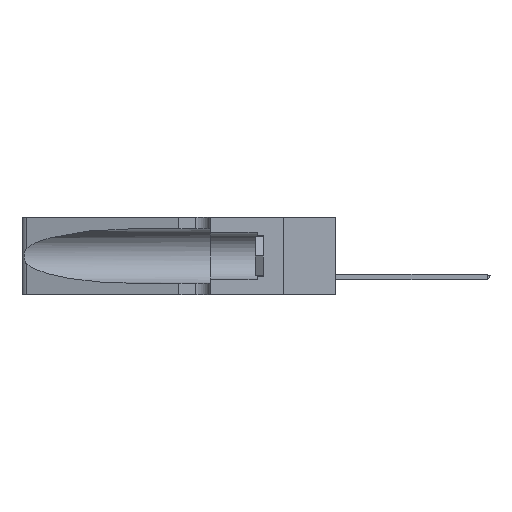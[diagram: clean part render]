
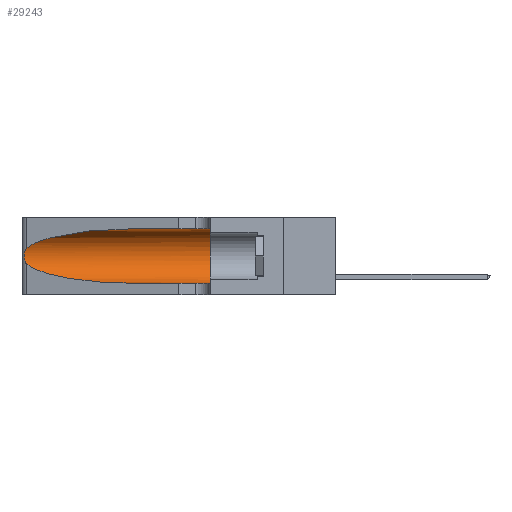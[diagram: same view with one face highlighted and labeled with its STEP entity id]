
A CAD part, left-side view. The second image highlights one B-rep face of the part: STEP entity #29243.
In plain terms, the highlighted cylindrical face has radius 3.308 mm (diameter 6.617 mm), a partial arc.
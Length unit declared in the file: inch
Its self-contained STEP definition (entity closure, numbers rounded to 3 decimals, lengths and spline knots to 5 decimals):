
#1858 = CARTESIAN_POINT ( 'NONE',  ( 0.25487, 1.22718, 0.22369 ) ) ;
#1922 = CARTESIAN_POINT ( 'NONE',  ( 0.2373, 1.15595, 0.08982 ) ) ;
#2333 = CARTESIAN_POINT ( 'NONE',  ( 0.1305, 0.72297, 0.05475 ) ) ;
#2973 = DIRECTION ( 'NONE',  ( 0., -1., 0. ) ) ;
#5405 = CARTESIAN_POINT ( 'NONE',  ( 0.25487, 1.22718, 0.14631 ) ) ;
#5697 = CARTESIAN_POINT ( 'NONE',  ( 0.25854, 1.2359, 0.20912 ) ) ;
#5818 = CIRCLE ( 'NONE', #12054, 0.13025 ) ;
#7218 = DIRECTION ( 'NONE',  ( 0., 0., 1. ) ) ;
#7239 = DIRECTION ( 'NONE',  ( 0., -1., 0. ) ) ;
#7393 = EDGE_CURVE ( 'NONE', #26052, #35483, #23787, .T. ) ;
#8834 = EDGE_CURVE ( 'NONE', #19129, #9179, #31826, .T. ) ;
#8883 = CARTESIAN_POINT ( 'NONE',  ( 0.26075, 1.23896, 0.178 ) ) ;
#9179 = VERTEX_POINT ( 'NONE', #26367 ) ;
#9189 = ORIENTED_EDGE ( 'NONE', *, *, #22624, .T. ) ;
#9213 = CARTESIAN_POINT ( 'NONE',  ( 0.1305, 1.61858, 0.31525 ) ) ;
#9993 = CARTESIAN_POINT ( 'NONE',  ( 0.1305, 0.35, 0.185 ) ) ;
#10041 = ORIENTED_EDGE ( 'NONE', *, *, #10810, .F. ) ;
#10499 = EDGE_LOOP ( 'NONE', ( #9189, #23590, #22509, #21826, #10041, #40537 ) ) ;
#10810 = EDGE_CURVE ( 'NONE', #35483, #9179, #5818, .T. ) ;
#11647 = AXIS2_PLACEMENT_3D ( 'NONE', #26036, #7239, #26172 ) ;
#12054 = AXIS2_PLACEMENT_3D ( 'NONE', #9993, #32404, #7218 ) ;
#12068 = CARTESIAN_POINT ( 'NONE',  ( 0.25487, 1.22718, 0.22369 ) ) ;
#12842 = CARTESIAN_POINT ( 'NONE',  ( 0.1305, 0.35, 0.31525 ) ) ;
#12976 = CARTESIAN_POINT ( 'NONE',  ( 0.25487, 1.22718, 0.22369 ) ) ;
#15399 = CARTESIAN_POINT ( 'NONE',  ( 0.25639, 1.23184, 0.21858 ) ) ;
#15544 = CARTESIAN_POINT ( 'NONE',  ( 0.25555, 1.22994, 0.2215 ) ) ;
#15869 = CARTESIAN_POINT ( 'NONE',  ( 0.1305, 1.61858, 0.05475 ) ) ;
#16660 = EDGE_CURVE ( 'NONE', #23271, #27142, #37375, .T. ) ;
#17278 = CARTESIAN_POINT ( 'NONE',  ( 0.1305, 0.72297, 0.31525 ) ) ;
#17687 = CARTESIAN_POINT ( 'NONE',  ( 0.2373, 1.15595, 0.28018 ) ) ;
#17763 = CARTESIAN_POINT ( 'NONE',  ( 0.25487, 1.22718, 0.14631 ) ) ;
#17846 = VECTOR ( 'NONE', #34708, 39.37008 ) ;
#18180 = CARTESIAN_POINT ( 'NONE',  ( 0.25787, 1.23484, 0.2124 ) ) ;
#18328 = CARTESIAN_POINT ( 'NONE',  ( 0.25856, 1.23593, 0.16098 ) ) ;
#18611 = CARTESIAN_POINT ( 'NONE',  ( 0.25487, 1.22718, 0.14631 ) ) ;
#19129 = VERTEX_POINT ( 'NONE', #24128 ) ;
#20222 = CARTESIAN_POINT ( 'NONE',  ( 0.1305, 0.72297, 0.31525 ) ) ;
#21520 = CARTESIAN_POINT ( 'NONE',  ( 0.25639, 1.23186, 0.15144 ) ) ;
#21826 = ORIENTED_EDGE ( 'NONE', *, *, #8834, .T. ) ;
#22342 = VECTOR ( 'NONE', #2973, 39.37008 ) ;
#22509 = ORIENTED_EDGE ( 'NONE', *, *, #26175, .T. ) ;
#22624 = EDGE_CURVE ( 'NONE', #26052, #23271, #36076, .T. ) ;
#23271 = VERTEX_POINT ( 'NONE', #12976 ) ;
#23590 = ORIENTED_EDGE ( 'NONE', *, *, #16660, .T. ) ;
#23787 = LINE ( 'NONE', #9213, #17846 ) ;
#23802 =( BOUNDED_CURVE ( )  B_SPLINE_CURVE ( 3, ( #5405, #1922, #34059, #2333 ),
 .UNSPECIFIED., .F., .T. ) 
 B_SPLINE_CURVE_WITH_KNOTS ( ( 4, 4 ),
 ( 3.44316, 4.71239 ),
 .UNSPECIFIED. ) 
 CURVE ( )  GEOMETRIC_REPRESENTATION_ITEM ( )  RATIONAL_B_SPLINE_CURVE ( ( 1., 0.87, 0.87, 1. ) ) 
 REPRESENTATION_ITEM ( '' )  );
#24128 = CARTESIAN_POINT ( 'NONE',  ( 0.1305, 0.72297, 0.05475 ) ) ;
#26036 = CARTESIAN_POINT ( 'NONE',  ( 0.1305, 1.61858, 0.185 ) ) ;
#26052 = VERTEX_POINT ( 'NONE', #20222 ) ;
#26172 = DIRECTION ( 'NONE',  ( 0., 0., -1. ) ) ;
#26175 = EDGE_CURVE ( 'NONE', #27142, #19129, #23802, .T. ) ;
#26367 = CARTESIAN_POINT ( 'NONE',  ( 0.1305, 0.35, 0.05475 ) ) ;
#27142 = VERTEX_POINT ( 'NONE', #17763 ) ;
#27181 = CARTESIAN_POINT ( 'NONE',  ( 0.18966, 0.96281, 0.31525 ) ) ;
#27805 = CARTESIAN_POINT ( 'NONE',  ( 0.26018, 1.23835, 0.19895 ) ) ;
#29243 = ADVANCED_FACE ( 'NONE', ( #38303 ), #31329, .F. ) ;
#30997 = CARTESIAN_POINT ( 'NONE',  ( 0.26075, 1.23896, 0.19203 ) ) ;
#31329 = CYLINDRICAL_SURFACE ( 'NONE', #11647, 0.13025 ) ;
#31826 = LINE ( 'NONE', #15869, #22342 ) ;
#32404 = DIRECTION ( 'NONE',  ( 0., 1., 0. ) ) ;
#34059 = CARTESIAN_POINT ( 'NONE',  ( 0.18966, 0.96281, 0.05475 ) ) ;
#34212 = CARTESIAN_POINT ( 'NONE',  ( 0.26017, 1.23833, 0.17102 ) ) ;
#34371 = CARTESIAN_POINT ( 'NONE',  ( 0.25555, 1.22993, 0.14849 ) ) ;
#34708 = DIRECTION ( 'NONE',  ( 0., -1., 0. ) ) ;
#35483 = VERTEX_POINT ( 'NONE', #12842 ) ;
#36076 =( BOUNDED_CURVE ( )  B_SPLINE_CURVE ( 3, ( #17278, #27181, #17687, #1858 ),
 .UNSPECIFIED., .F., .F. ) 
 B_SPLINE_CURVE_WITH_KNOTS ( ( 4, 4 ),
 ( 1.5708, 2.84003 ),
 .UNSPECIFIED. ) 
 CURVE ( )  GEOMETRIC_REPRESENTATION_ITEM ( )  RATIONAL_B_SPLINE_CURVE ( ( 1., 0.87, 0.87, 1. ) ) 
 REPRESENTATION_ITEM ( '' )  );
#37375 = B_SPLINE_CURVE_WITH_KNOTS ( 'NONE', 3,
 ( #12068, #15544, #15399, #18180, #5697, #27805, #30997, #8883, #34212, #18328, #40582, #21520, #34371, #18611 ),
 .UNSPECIFIED., .F., .F.,
 ( 4, 2, 2, 2, 2, 2, 4 ),
 ( 0., 0.00027, 0.00053, 0.00107, 0.0016, 0.00187, 0.00214 ),
 .UNSPECIFIED. ) ;
#38303 = FACE_OUTER_BOUND ( 'NONE', #10499, .T. ) ;
#40537 = ORIENTED_EDGE ( 'NONE', *, *, #7393, .F. ) ;
#40582 = CARTESIAN_POINT ( 'NONE',  ( 0.25789, 1.23486, 0.15765 ) ) ;
